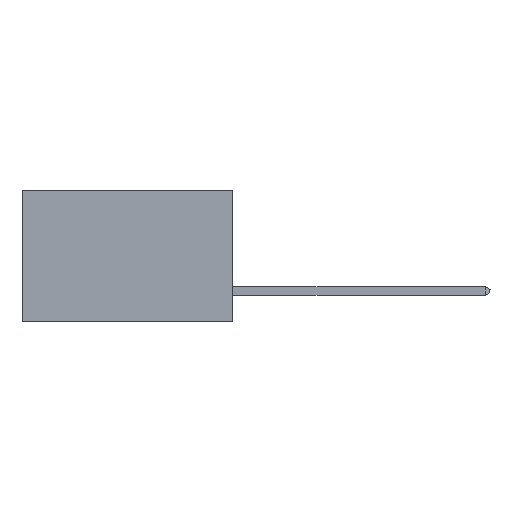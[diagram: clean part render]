
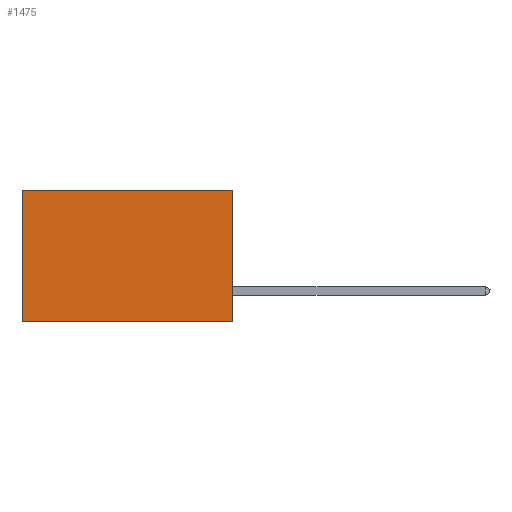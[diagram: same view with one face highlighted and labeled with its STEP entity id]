
A CAD part, left-side view. The second image highlights one B-rep face of the part: STEP entity #1475.
In plain terms, the highlighted planar face has unit normal (-1, 0, 0).
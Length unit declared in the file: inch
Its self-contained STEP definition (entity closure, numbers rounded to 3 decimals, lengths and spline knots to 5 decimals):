
#495 = LINE ( 'NONE', #3894, #4693 ) ;
#654 = DIRECTION ( 'NONE',  ( 0., 0., -1. ) ) ;
#1128 = VECTOR ( 'NONE', #9523, 39.37008 ) ;
#1475 = ADVANCED_FACE ( 'NONE', ( #11038 ), #17592, .F. ) ;
#1683 = DIRECTION ( 'NONE',  ( 1., 0., 0. ) ) ;
#2290 = ORIENTED_EDGE ( 'NONE', *, *, #4543, .F. ) ;
#2523 = VECTOR ( 'NONE', #16275, 39.37008 ) ;
#2604 = LINE ( 'NONE', #14053, #1128 ) ;
#3308 = CARTESIAN_POINT ( 'NONE',  ( 0.2875, 0., -0.375 ) ) ;
#3542 = CARTESIAN_POINT ( 'NONE',  ( 0.2875, 0.6, -0.375 ) ) ;
#3887 = CARTESIAN_POINT ( 'NONE',  ( 0.2875, 0.6, 0. ) ) ;
#3894 = CARTESIAN_POINT ( 'NONE',  ( 0.2875, 0., -0.375 ) ) ;
#4464 = VERTEX_POINT ( 'NONE', #3542 ) ;
#4543 = EDGE_CURVE ( 'NONE', #17568, #5135, #495, .T. ) ;
#4693 = VECTOR ( 'NONE', #654, 39.37008 ) ;
#4834 = ORIENTED_EDGE ( 'NONE', *, *, #18370, .T. ) ;
#5135 = VERTEX_POINT ( 'NONE', #10958 ) ;
#5395 = ORIENTED_EDGE ( 'NONE', *, *, #14155, .T. ) ;
#5399 = CARTESIAN_POINT ( 'NONE',  ( 0.2875, 0., 0. ) ) ;
#5597 = LINE ( 'NONE', #8723, #20276 ) ;
#6381 = VERTEX_POINT ( 'NONE', #3887 ) ;
#6761 = AXIS2_PLACEMENT_3D ( 'NONE', #3308, #1683, #11095 ) ;
#7115 = DIRECTION ( 'NONE',  ( 0., 0., -1. ) ) ;
#7701 = EDGE_LOOP ( 'NONE', ( #4834, #7818, #2290, #5395 ) ) ;
#7818 = ORIENTED_EDGE ( 'NONE', *, *, #18573, .F. ) ;
#8723 = CARTESIAN_POINT ( 'NONE',  ( 0.2875, 0.6, -0.375 ) ) ;
#8763 = LINE ( 'NONE', #14674, #2523 ) ;
#9523 = DIRECTION ( 'NONE',  ( 0., 1., 0. ) ) ;
#10958 = CARTESIAN_POINT ( 'NONE',  ( 0.2875, 0., -0.375 ) ) ;
#11038 = FACE_OUTER_BOUND ( 'NONE', #7701, .T. ) ;
#11095 = DIRECTION ( 'NONE',  ( 0., 0., -1. ) ) ;
#14053 = CARTESIAN_POINT ( 'NONE',  ( 0.2875, 0., -0.375 ) ) ;
#14155 = EDGE_CURVE ( 'NONE', #17568, #6381, #8763, .T. ) ;
#14674 = CARTESIAN_POINT ( 'NONE',  ( 0.2875, 0., 0. ) ) ;
#16275 = DIRECTION ( 'NONE',  ( 0., 1., 0. ) ) ;
#17568 = VERTEX_POINT ( 'NONE', #5399 ) ;
#17592 = PLANE ( 'NONE',  #6761 ) ;
#18370 = EDGE_CURVE ( 'NONE', #6381, #4464, #5597, .T. ) ;
#18573 = EDGE_CURVE ( 'NONE', #5135, #4464, #2604, .T. ) ;
#20276 = VECTOR ( 'NONE', #7115, 39.37008 ) ;
